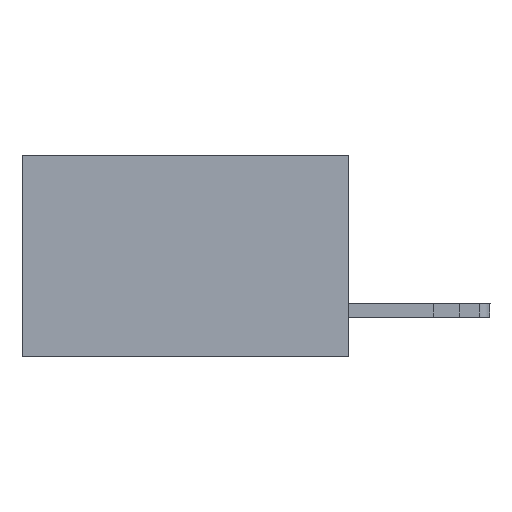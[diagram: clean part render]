
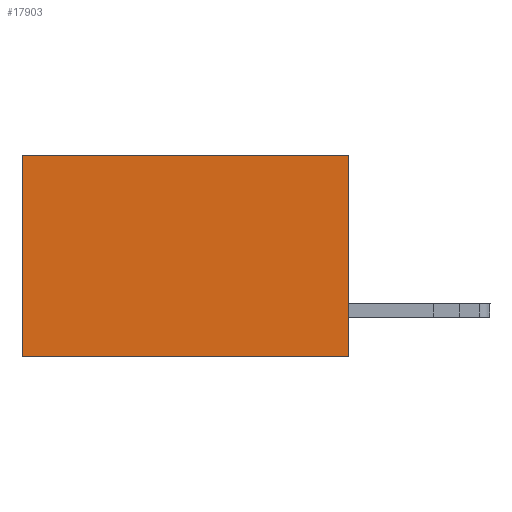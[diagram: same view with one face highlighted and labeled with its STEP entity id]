
A CAD part, left-side view. The second image highlights one B-rep face of the part: STEP entity #17903.
In plain terms, the highlighted planar face has unit normal (-1, 0, 0).
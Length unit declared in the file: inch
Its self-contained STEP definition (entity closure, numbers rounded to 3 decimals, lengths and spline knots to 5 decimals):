
#190 = CARTESIAN_POINT ( 'NONE',  ( 0.2615, 0.6, -0.37 ) ) ;
#417 = VECTOR ( 'NONE', #17229, 39.37008 ) ;
#1850 = VECTOR ( 'NONE', #14209, 39.37008 ) ;
#2725 = ORIENTED_EDGE ( 'NONE', *, *, #15660, .T. ) ;
#5383 = DIRECTION ( 'NONE',  ( 0., 0., -1. ) ) ;
#5450 = DIRECTION ( 'NONE',  ( 1., 0., 0. ) ) ;
#5468 = CARTESIAN_POINT ( 'NONE',  ( 0.2615, 0., -0.37 ) ) ;
#5651 = VERTEX_POINT ( 'NONE', #16871 ) ;
#5798 = PLANE ( 'NONE',  #7885 ) ;
#7789 = DIRECTION ( 'NONE',  ( 0., 1., 0. ) ) ;
#7885 = AXIS2_PLACEMENT_3D ( 'NONE', #5468, #5450, #5383 ) ;
#7895 = ORIENTED_EDGE ( 'NONE', *, *, #9417, .T. ) ;
#8273 = FACE_OUTER_BOUND ( 'NONE', #20664, .T. ) ;
#8523 = ORIENTED_EDGE ( 'NONE', *, *, #11621, .F. ) ;
#9065 = CARTESIAN_POINT ( 'NONE',  ( 0.2615, 0.6, 0. ) ) ;
#9417 = EDGE_CURVE ( 'NONE', #15621, #10085, #9642, .T. ) ;
#9642 = LINE ( 'NONE', #17048, #417 ) ;
#10085 = VERTEX_POINT ( 'NONE', #9065 ) ;
#10594 = ORIENTED_EDGE ( 'NONE', *, *, #17752, .F. ) ;
#11542 = LINE ( 'NONE', #15680, #1850 ) ;
#11621 = EDGE_CURVE ( 'NONE', #15621, #5651, #21332, .T. ) ;
#12454 = CARTESIAN_POINT ( 'NONE',  ( 0.2615, 0., 0. ) ) ;
#13509 = VECTOR ( 'NONE', #7789, 39.37008 ) ;
#14209 = DIRECTION ( 'NONE',  ( 0., 0., -1. ) ) ;
#15621 = VERTEX_POINT ( 'NONE', #12454 ) ;
#15660 = EDGE_CURVE ( 'NONE', #10085, #19260, #11542, .T. ) ;
#15680 = CARTESIAN_POINT ( 'NONE',  ( 0.2615, 0.6, -0.37 ) ) ;
#16274 = CARTESIAN_POINT ( 'NONE',  ( 0.2615, 0., -0.37 ) ) ;
#16871 = CARTESIAN_POINT ( 'NONE',  ( 0.2615, 0., -0.37 ) ) ;
#16993 = VECTOR ( 'NONE', #19763, 39.37008 ) ;
#17048 = CARTESIAN_POINT ( 'NONE',  ( 0.2615, 0., 0. ) ) ;
#17229 = DIRECTION ( 'NONE',  ( 0., 1., 0. ) ) ;
#17752 = EDGE_CURVE ( 'NONE', #5651, #19260, #18030, .T. ) ;
#17903 = ADVANCED_FACE ( 'NONE', ( #8273 ), #5798, .F. ) ;
#18030 = LINE ( 'NONE', #16274, #13509 ) ;
#19260 = VERTEX_POINT ( 'NONE', #190 ) ;
#19763 = DIRECTION ( 'NONE',  ( 0., 0., -1. ) ) ;
#20235 = CARTESIAN_POINT ( 'NONE',  ( 0.2615, 0., -0.37 ) ) ;
#20664 = EDGE_LOOP ( 'NONE', ( #2725, #10594, #8523, #7895 ) ) ;
#21332 = LINE ( 'NONE', #20235, #16993 ) ;
